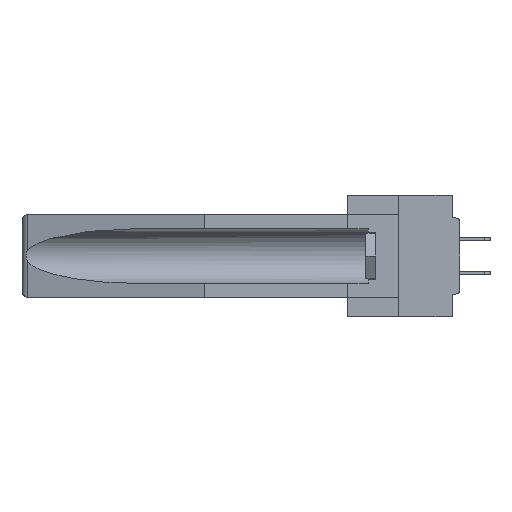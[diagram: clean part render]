
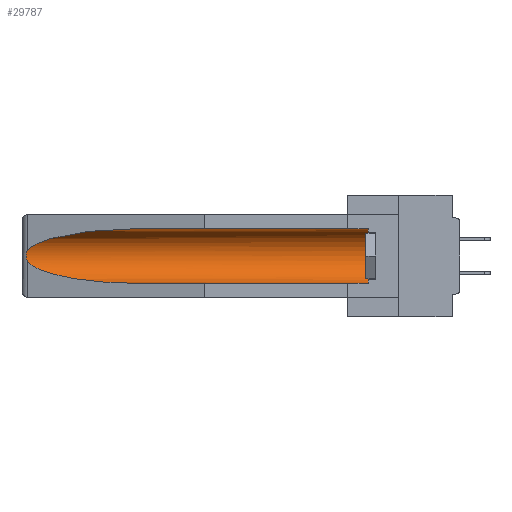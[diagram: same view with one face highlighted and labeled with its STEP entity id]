
A CAD part, left-side view. The second image highlights one B-rep face of the part: STEP entity #29787.
In plain terms, the highlighted cylindrical face has radius 2.857 mm (diameter 5.715 mm), a partial arc.
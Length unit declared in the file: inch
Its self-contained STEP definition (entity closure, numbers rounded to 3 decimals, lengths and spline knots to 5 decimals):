
#322 = CIRCLE ( 'NONE', #33774, 0.1125 ) ;
#509 =( BOUNDED_CURVE ( )  B_SPLINE_CURVE ( 3, ( #10087, #21968, #7067, #37219 ),
 .UNSPECIFIED., .F., .F. ) 
 B_SPLINE_CURVE_WITH_KNOTS ( ( 4, 4 ),
 ( 4.71239, 6.08839 ),
 .UNSPECIFIED. ) 
 CURVE ( )  GEOMETRIC_REPRESENTATION_ITEM ( )  RATIONAL_B_SPLINE_CURVE ( ( 1., 0.848, 0.848, 1. ) ) 
 REPRESENTATION_ITEM ( '' )  );
#563 = CARTESIAN_POINT ( 'NONE',  ( 0.2675, 1.53308, -0.17534 ) ) ;
#770 = VERTEX_POINT ( 'NONE', #6973 ) ;
#1667 = VERTEX_POINT ( 'NONE', #35398 ) ;
#1747 = CARTESIAN_POINT ( 'NONE',  ( 0.155, -0.30754, -0.1715 ) ) ;
#2182 =( BOUNDED_CURVE ( )  B_SPLINE_CURVE ( 3, ( #2565, #5436, #38912, #11831 ),
 .UNSPECIFIED., .F., .F. ) 
 B_SPLINE_CURVE_WITH_KNOTS ( ( 4, 4 ),
 ( 0.1948, 1.5708 ),
 .UNSPECIFIED. ) 
 CURVE ( )  GEOMETRIC_REPRESENTATION_ITEM ( )  RATIONAL_B_SPLINE_CURVE ( ( 1., 0.848, 0.848, 1. ) ) 
 REPRESENTATION_ITEM ( '' )  );
#2565 = CARTESIAN_POINT ( 'NONE',  ( 0.26537, 1.52718, -0.19328 ) ) ;
#2659 = CARTESIAN_POINT ( 'NONE',  ( 0.155, 1.07973, -0.284 ) ) ;
#3568 = CARTESIAN_POINT ( 'NONE',  ( 0.26537, 1.52718, -0.19328 ) ) ;
#3613 = EDGE_CURVE ( 'NONE', #1667, #14131, #2182, .T. ) ;
#3622 = CARTESIAN_POINT ( 'NONE',  ( 0.155, 0.126, -0.1715 ) ) ;
#4111 = FACE_OUTER_BOUND ( 'NONE', #31896, .T. ) ;
#5391 = CARTESIAN_POINT ( 'NONE',  ( 0.155, 0.126, -0.059 ) ) ;
#5436 = CARTESIAN_POINT ( 'NONE',  ( 0.25451, 1.48313, -0.24835 ) ) ;
#5994 = CYLINDRICAL_SURFACE ( 'NONE', #6424, 0.1125 ) ;
#5995 = LINE ( 'NONE', #17963, #31146 ) ;
#6424 = AXIS2_PLACEMENT_3D ( 'NONE', #1747, #17266, #8604 ) ;
#6973 = CARTESIAN_POINT ( 'NONE',  ( 0.26537, 1.52718, -0.14972 ) ) ;
#7067 = CARTESIAN_POINT ( 'NONE',  ( 0.25451, 1.48313, -0.09465 ) ) ;
#7740 = EDGE_CURVE ( 'NONE', #12188, #14131, #5995, .T. ) ;
#8604 = DIRECTION ( 'NONE',  ( 0., 0., 1. ) ) ;
#9011 = CARTESIAN_POINT ( 'NONE',  ( 0.26654, 1.53092, -0.15636 ) ) ;
#9138 = CARTESIAN_POINT ( 'NONE',  ( 0.2675, 1.53308, -0.16763 ) ) ;
#9767 = EDGE_CURVE ( 'NONE', #770, #1667, #12147, .T. ) ;
#10087 = CARTESIAN_POINT ( 'NONE',  ( 0.155, 1.07973, -0.059 ) ) ;
#11831 = CARTESIAN_POINT ( 'NONE',  ( 0.155, 1.07973, -0.284 ) ) ;
#12147 = B_SPLINE_CURVE_WITH_KNOTS ( 'NONE', 3,
 ( #15127, #33378, #9011, #33508, #9138, #563, #15534, #15666, #15266, #3568 ),
 .UNSPECIFIED., .F., .F.,
 ( 4, 2, 2, 2, 4 ),
 ( 0., 0.00029, 0.00058, 0.00087, 0.00117 ),
 .UNSPECIFIED. ) ;
#12188 = VERTEX_POINT ( 'NONE', #23682 ) ;
#14131 = VERTEX_POINT ( 'NONE', #2659 ) ;
#15127 = CARTESIAN_POINT ( 'NONE',  ( 0.26537, 1.52718, -0.14972 ) ) ;
#15266 = CARTESIAN_POINT ( 'NONE',  ( 0.26597, 1.5296, -0.19026 ) ) ;
#15534 = CARTESIAN_POINT ( 'NONE',  ( 0.2673, 1.53269, -0.17917 ) ) ;
#15666 = CARTESIAN_POINT ( 'NONE',  ( 0.26655, 1.53094, -0.18657 ) ) ;
#16953 = CARTESIAN_POINT ( 'NONE',  ( 0.155, 1.07973, -0.059 ) ) ;
#17011 = ORIENTED_EDGE ( 'NONE', *, *, #28503, .T. ) ;
#17266 = DIRECTION ( 'NONE',  ( 0., 1., 0. ) ) ;
#17963 = CARTESIAN_POINT ( 'NONE',  ( 0.155, -0.30754, -0.284 ) ) ;
#19021 = ORIENTED_EDGE ( 'NONE', *, *, #3613, .T. ) ;
#20166 = VERTEX_POINT ( 'NONE', #5391 ) ;
#21139 = DIRECTION ( 'NONE',  ( 0., 1., 0. ) ) ;
#21968 = CARTESIAN_POINT ( 'NONE',  ( 0.21114, 1.30732, -0.059 ) ) ;
#23682 = CARTESIAN_POINT ( 'NONE',  ( 0.155, 0.126, -0.284 ) ) ;
#24044 = ORIENTED_EDGE ( 'NONE', *, *, #9767, .T. ) ;
#24859 = DIRECTION ( 'NONE',  ( 0., -1., 0. ) ) ;
#25269 = ORIENTED_EDGE ( 'NONE', *, *, #31775, .T. ) ;
#27707 = ORIENTED_EDGE ( 'NONE', *, *, #7740, .F. ) ;
#28170 = DIRECTION ( 'NONE',  ( 0., 0., 1. ) ) ;
#28435 = LINE ( 'NONE', #29988, #33146 ) ;
#28503 = EDGE_CURVE ( 'NONE', #20166, #30252, #28435, .T. ) ;
#29787 = ADVANCED_FACE ( 'NONE', ( #4111 ), #5994, .F. ) ;
#29988 = CARTESIAN_POINT ( 'NONE',  ( 0.155, -0.30754, -0.059 ) ) ;
#30252 = VERTEX_POINT ( 'NONE', #16953 ) ;
#31146 = VECTOR ( 'NONE', #21139, 39.37008 ) ;
#31775 = EDGE_CURVE ( 'NONE', #30252, #770, #509, .T. ) ;
#31896 = EDGE_LOOP ( 'NONE', ( #25269, #24044, #19021, #27707, #32572, #17011 ) ) ;
#32572 = ORIENTED_EDGE ( 'NONE', *, *, #36042, .T. ) ;
#33146 = VECTOR ( 'NONE', #36142, 39.37008 ) ;
#33378 = CARTESIAN_POINT ( 'NONE',  ( 0.26597, 1.52961, -0.15275 ) ) ;
#33508 = CARTESIAN_POINT ( 'NONE',  ( 0.2673, 1.5327, -0.16383 ) ) ;
#33774 = AXIS2_PLACEMENT_3D ( 'NONE', #3622, #24859, #28170 ) ;
#35398 = CARTESIAN_POINT ( 'NONE',  ( 0.26537, 1.52718, -0.19328 ) ) ;
#36042 = EDGE_CURVE ( 'NONE', #12188, #20166, #322, .T. ) ;
#36142 = DIRECTION ( 'NONE',  ( 0., 1., 0. ) ) ;
#37219 = CARTESIAN_POINT ( 'NONE',  ( 0.26537, 1.52718, -0.14972 ) ) ;
#38912 = CARTESIAN_POINT ( 'NONE',  ( 0.21114, 1.30732, -0.284 ) ) ;
